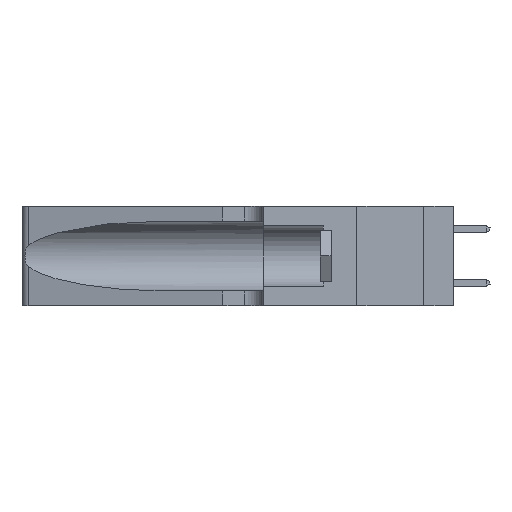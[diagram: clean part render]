
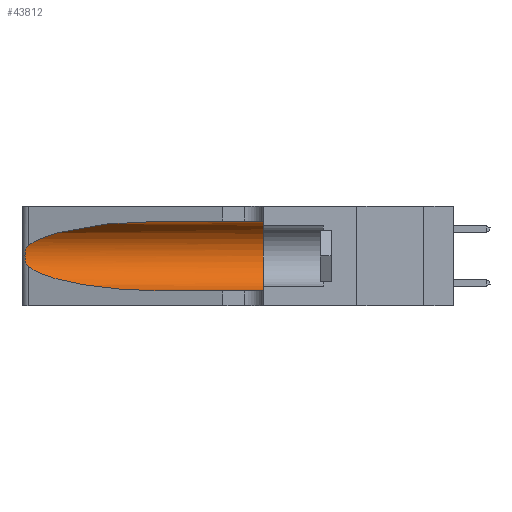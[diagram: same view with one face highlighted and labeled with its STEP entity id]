
A CAD part, left-side view. The second image highlights one B-rep face of the part: STEP entity #43812.
In plain terms, the highlighted cylindrical face has radius 3.308 mm (diameter 6.617 mm), a partial arc.
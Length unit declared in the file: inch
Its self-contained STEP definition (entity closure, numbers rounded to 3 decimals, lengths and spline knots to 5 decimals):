
#555 = CARTESIAN_POINT ( 'NONE',  ( 0.1305, 0.35, 0.05475 ) ) ;
#1473 = CARTESIAN_POINT ( 'NONE',  ( 0.25487, 1.22718, 0.14631 ) ) ;
#2569 = CARTESIAN_POINT ( 'NONE',  ( 0.26018, 1.23835, 0.19895 ) ) ;
#4151 = VERTEX_POINT ( 'NONE', #20992 ) ;
#4713 = CARTESIAN_POINT ( 'NONE',  ( 0.1305, 1.61858, 0.05475 ) ) ;
#5124 = CARTESIAN_POINT ( 'NONE',  ( 0.2373, 1.15595, 0.08982 ) ) ;
#6180 = CARTESIAN_POINT ( 'NONE',  ( 0.26075, 1.23896, 0.178 ) ) ;
#6575 = EDGE_CURVE ( 'NONE', #4151, #37700, #20191, .T. ) ;
#6703 = DIRECTION ( 'NONE',  ( 0., 0., -1. ) ) ;
#7222 =( BOUNDED_CURVE ( )  B_SPLINE_CURVE ( 3, ( #1473, #5124, #8709, #33749 ),
 .UNSPECIFIED., .F., .T. ) 
 B_SPLINE_CURVE_WITH_KNOTS ( ( 4, 4 ),
 ( 3.44316, 4.71239 ),
 .UNSPECIFIED. ) 
 CURVE ( )  GEOMETRIC_REPRESENTATION_ITEM ( )  RATIONAL_B_SPLINE_CURVE ( ( 1., 0.87, 0.87, 1. ) ) 
 REPRESENTATION_ITEM ( '' )  );
#7610 = CARTESIAN_POINT ( 'NONE',  ( 0.18966, 0.96281, 0.31525 ) ) ;
#8490 = CARTESIAN_POINT ( 'NONE',  ( 0.1305, 0.35, 0.31525 ) ) ;
#8656 = LINE ( 'NONE', #44588, #27759 ) ;
#8709 = CARTESIAN_POINT ( 'NONE',  ( 0.18966, 0.96281, 0.05475 ) ) ;
#9799 = CARTESIAN_POINT ( 'NONE',  ( 0.25856, 1.23593, 0.16098 ) ) ;
#10621 = VECTOR ( 'NONE', #11888, 39.37008 ) ;
#10657 = B_SPLINE_CURVE_WITH_KNOTS ( 'NONE', 3,
 ( #38280, #41813, #20468, #45376, #24074, #2569, #27703, #6180, #31264, #9799, #34851, #13372, #38426, #17031 ),
 .UNSPECIFIED., .F., .F.,
 ( 4, 2, 2, 2, 2, 2, 4 ),
 ( 0., 0.00027, 0.00053, 0.00107, 0.0016, 0.00187, 0.00214 ),
 .UNSPECIFIED. ) ;
#11208 = CARTESIAN_POINT ( 'NONE',  ( 0.2373, 1.15595, 0.28018 ) ) ;
#11888 = DIRECTION ( 'NONE',  ( 0., -1., 0. ) ) ;
#11934 = DIRECTION ( 'NONE',  ( 0., 1., 0. ) ) ;
#12830 = ORIENTED_EDGE ( 'NONE', *, *, #31506, .T. ) ;
#13107 = EDGE_LOOP ( 'NONE', ( #25928, #12830, #38304, #14525, #21141, #19349 ) ) ;
#13372 = CARTESIAN_POINT ( 'NONE',  ( 0.25639, 1.23186, 0.15144 ) ) ;
#13883 = DIRECTION ( 'NONE',  ( 0., -1., 0. ) ) ;
#14525 = ORIENTED_EDGE ( 'NONE', *, *, #6575, .T. ) ;
#15598 = AXIS2_PLACEMENT_3D ( 'NONE', #31781, #13883, #6703 ) ;
#16080 = DIRECTION ( 'NONE',  ( 0., -1., 0. ) ) ;
#17031 = CARTESIAN_POINT ( 'NONE',  ( 0.25487, 1.22718, 0.14631 ) ) ;
#18773 = EDGE_CURVE ( 'NONE', #23189, #21855, #27390, .T. ) ;
#19349 = ORIENTED_EDGE ( 'NONE', *, *, #40782, .F. ) ;
#20191 = LINE ( 'NONE', #4713, #10621 ) ;
#20468 = CARTESIAN_POINT ( 'NONE',  ( 0.25639, 1.23184, 0.21858 ) ) ;
#20927 = EDGE_CURVE ( 'NONE', #33101, #37700, #42845, .T. ) ;
#20992 = CARTESIAN_POINT ( 'NONE',  ( 0.1305, 0.72297, 0.05475 ) ) ;
#21098 = VERTEX_POINT ( 'NONE', #34188 ) ;
#21141 = ORIENTED_EDGE ( 'NONE', *, *, #20927, .F. ) ;
#21855 = VERTEX_POINT ( 'NONE', #45266 ) ;
#23189 = VERTEX_POINT ( 'NONE', #37450 ) ;
#24074 = CARTESIAN_POINT ( 'NONE',  ( 0.25854, 1.2359, 0.20912 ) ) ;
#25928 = ORIENTED_EDGE ( 'NONE', *, *, #18773, .T. ) ;
#26111 = AXIS2_PLACEMENT_3D ( 'NONE', #33400, #11934, #36997 ) ;
#26465 = FACE_OUTER_BOUND ( 'NONE', #13107, .T. ) ;
#27390 =( BOUNDED_CURVE ( )  B_SPLINE_CURVE ( 3, ( #32678, #7610, #11208, #36278 ),
 .UNSPECIFIED., .F., .F. ) 
 B_SPLINE_CURVE_WITH_KNOTS ( ( 4, 4 ),
 ( 1.5708, 2.84003 ),
 .UNSPECIFIED. ) 
 CURVE ( )  GEOMETRIC_REPRESENTATION_ITEM ( )  RATIONAL_B_SPLINE_CURVE ( ( 1., 0.87, 0.87, 1. ) ) 
 REPRESENTATION_ITEM ( '' )  );
#27703 = CARTESIAN_POINT ( 'NONE',  ( 0.26075, 1.23896, 0.19203 ) ) ;
#27759 = VECTOR ( 'NONE', #16080, 39.37008 ) ;
#31264 = CARTESIAN_POINT ( 'NONE',  ( 0.26017, 1.23833, 0.17102 ) ) ;
#31506 = EDGE_CURVE ( 'NONE', #21855, #21098, #10657, .T. ) ;
#31781 = CARTESIAN_POINT ( 'NONE',  ( 0.1305, 1.61858, 0.185 ) ) ;
#32678 = CARTESIAN_POINT ( 'NONE',  ( 0.1305, 0.72297, 0.31525 ) ) ;
#33101 = VERTEX_POINT ( 'NONE', #8490 ) ;
#33400 = CARTESIAN_POINT ( 'NONE',  ( 0.1305, 0.35, 0.185 ) ) ;
#33664 = CYLINDRICAL_SURFACE ( 'NONE', #15598, 0.13025 ) ;
#33749 = CARTESIAN_POINT ( 'NONE',  ( 0.1305, 0.72297, 0.05475 ) ) ;
#34188 = CARTESIAN_POINT ( 'NONE',  ( 0.25487, 1.22718, 0.14631 ) ) ;
#34851 = CARTESIAN_POINT ( 'NONE',  ( 0.25789, 1.23486, 0.15765 ) ) ;
#36278 = CARTESIAN_POINT ( 'NONE',  ( 0.25487, 1.22718, 0.22369 ) ) ;
#36997 = DIRECTION ( 'NONE',  ( 0., 0., 1. ) ) ;
#37450 = CARTESIAN_POINT ( 'NONE',  ( 0.1305, 0.72297, 0.31525 ) ) ;
#37700 = VERTEX_POINT ( 'NONE', #555 ) ;
#38280 = CARTESIAN_POINT ( 'NONE',  ( 0.25487, 1.22718, 0.22369 ) ) ;
#38304 = ORIENTED_EDGE ( 'NONE', *, *, #46302, .T. ) ;
#38426 = CARTESIAN_POINT ( 'NONE',  ( 0.25555, 1.22993, 0.14849 ) ) ;
#40782 = EDGE_CURVE ( 'NONE', #23189, #33101, #8656, .T. ) ;
#41813 = CARTESIAN_POINT ( 'NONE',  ( 0.25555, 1.22994, 0.2215 ) ) ;
#42845 = CIRCLE ( 'NONE', #26111, 0.13025 ) ;
#43812 = ADVANCED_FACE ( 'NONE', ( #26465 ), #33664, .F. ) ;
#44588 = CARTESIAN_POINT ( 'NONE',  ( 0.1305, 1.61858, 0.31525 ) ) ;
#45266 = CARTESIAN_POINT ( 'NONE',  ( 0.25487, 1.22718, 0.22369 ) ) ;
#45376 = CARTESIAN_POINT ( 'NONE',  ( 0.25787, 1.23484, 0.2124 ) ) ;
#46302 = EDGE_CURVE ( 'NONE', #21098, #4151, #7222, .T. ) ;
